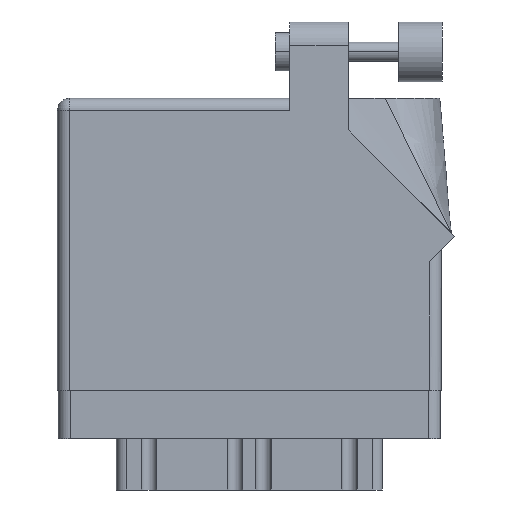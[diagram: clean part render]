
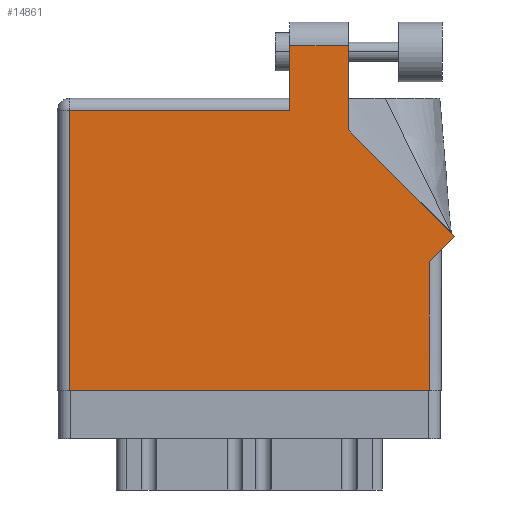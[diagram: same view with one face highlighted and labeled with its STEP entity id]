
A CAD part, front view. The second image highlights one B-rep face of the part: STEP entity #14861.
In plain terms, the highlighted face is planar.
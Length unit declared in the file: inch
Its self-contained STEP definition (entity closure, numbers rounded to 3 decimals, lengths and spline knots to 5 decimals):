
#793 = ORIENTED_EDGE ( 'NONE', *, *, #37293, .T. ) ;
#1068 = VECTOR ( 'NONE', #19315, 39.37008 ) ;
#1271 = PLANE ( 'NONE',  #6959 ) ;
#2713 = VECTOR ( 'NONE', #18833, 39.37008 ) ;
#2743 = CARTESIAN_POINT ( 'NONE',  ( 0.062, 0., 0. ) ) ;
#2892 = CARTESIAN_POINT ( 'NONE',  ( 1.948, 0., 0. ) ) ;
#3234 = VERTEX_POINT ( 'NONE', #12394 ) ;
#3263 = DIRECTION ( 'NONE',  ( -1., 0., 0. ) ) ;
#3584 = VECTOR ( 'NONE', #3263, 39.37008 ) ;
#3685 = EDGE_CURVE ( 'NONE', #7406, #26864, #22267, .T. ) ;
#4412 = CARTESIAN_POINT ( 'NONE',  ( 2.08071, 0.80771, 0. ) ) ;
#4518 = LINE ( 'NONE', #28428, #2713 ) ;
#6959 = AXIS2_PLACEMENT_3D ( 'NONE', #7171, #9752, #21686 ) ;
#6985 = CARTESIAN_POINT ( 'NONE',  ( 1.524, 1.805, 0. ) ) ;
#7171 = CARTESIAN_POINT ( 'NONE',  ( 0., 1.53, 0. ) ) ;
#7406 = VERTEX_POINT ( 'NONE', #2892 ) ;
#7435 = EDGE_CURVE ( 'NONE', #16643, #3234, #27183, .T. ) ;
#9401 = DIRECTION ( 'NONE',  ( 0., -1., 0. ) ) ;
#9676 = VERTEX_POINT ( 'NONE', #10788 ) ;
#9752 = DIRECTION ( 'NONE',  ( 0., 0., -1. ) ) ;
#9980 = EDGE_CURVE ( 'NONE', #36899, #30317, #17829, .T. ) ;
#10038 = ORIENTED_EDGE ( 'NONE', *, *, #17432, .T. ) ;
#10179 = VECTOR ( 'NONE', #17977, 39.37008 ) ;
#10788 = CARTESIAN_POINT ( 'NONE',  ( 2.08071, 0.80771, 0. ) ) ;
#11109 = CARTESIAN_POINT ( 'NONE',  ( 1.948, 0.737, 0. ) ) ;
#11259 = EDGE_CURVE ( 'NONE', #3234, #19204, #32910, .T. ) ;
#11352 = VECTOR ( 'NONE', #29773, 39.37008 ) ;
#11795 = CARTESIAN_POINT ( 'NONE',  ( 1.217, 1.468, 0. ) ) ;
#12394 = CARTESIAN_POINT ( 'NONE',  ( 0.062, 1.468, 0. ) ) ;
#12855 = LINE ( 'NONE', #4412, #1068 ) ;
#13798 = VECTOR ( 'NONE', #32057, 39.37008 ) ;
#14247 = EDGE_CURVE ( 'NONE', #30317, #24032, #20566, .T. ) ;
#14861 = ADVANCED_FACE ( 'NONE', ( #21871 ), #1271, .F. ) ;
#16643 = VERTEX_POINT ( 'NONE', #11795 ) ;
#16920 = EDGE_CURVE ( 'NONE', #26864, #9676, #32847, .T. ) ;
#17141 = VECTOR ( 'NONE', #17505, 39.37008 ) ;
#17432 = EDGE_CURVE ( 'NONE', #19204, #7406, #4518, .T. ) ;
#17505 = DIRECTION ( 'NONE',  ( 0., -1., 0. ) ) ;
#17627 = CARTESIAN_POINT ( 'NONE',  ( 1.217, 1.805, 0. ) ) ;
#17829 = LINE ( 'NONE', #21326, #11352 ) ;
#17896 = LINE ( 'NONE', #36609, #17141 ) ;
#17977 = DIRECTION ( 'NONE',  ( 0.707, 0.707, 0. ) ) ;
#17988 = CARTESIAN_POINT ( 'NONE',  ( 0., 1.468, 0. ) ) ;
#18727 = VECTOR ( 'NONE', #9401, 39.37008 ) ;
#18833 = DIRECTION ( 'NONE',  ( 1., 0., 0. ) ) ;
#19204 = VERTEX_POINT ( 'NONE', #28458 ) ;
#19315 = DIRECTION ( 'NONE',  ( -0.707, 0.707, 0. ) ) ;
#19731 = ORIENTED_EDGE ( 'NONE', *, *, #9980, .T. ) ;
#19830 = VECTOR ( 'NONE', #29573, 39.37008 ) ;
#20566 = LINE ( 'NONE', #17627, #19830 ) ;
#21326 = CARTESIAN_POINT ( 'NONE',  ( 1.524, 1.36442, 0. ) ) ;
#21686 = DIRECTION ( 'NONE',  ( -1., 0., 0. ) ) ;
#21871 = FACE_OUTER_BOUND ( 'NONE', #36660, .T. ) ;
#22267 = LINE ( 'NONE', #11109, #13798 ) ;
#22998 = CARTESIAN_POINT ( 'NONE',  ( 1.217, 1.805, 0. ) ) ;
#24032 = VERTEX_POINT ( 'NONE', #22998 ) ;
#24118 = EDGE_CURVE ( 'NONE', #24032, #16643, #17896, .T. ) ;
#24464 = CARTESIAN_POINT ( 'NONE',  ( 1.524, 1.36442, 0. ) ) ;
#24467 = ORIENTED_EDGE ( 'NONE', *, *, #16920, .T. ) ;
#26864 = VERTEX_POINT ( 'NONE', #31203 ) ;
#27183 = LINE ( 'NONE', #17988, #3584 ) ;
#28428 = CARTESIAN_POINT ( 'NONE',  ( 0., 0., 0. ) ) ;
#28458 = CARTESIAN_POINT ( 'NONE',  ( 0.062, 0., 0. ) ) ;
#29552 = ORIENTED_EDGE ( 'NONE', *, *, #7435, .T. ) ;
#29573 = DIRECTION ( 'NONE',  ( -1., 0., 0. ) ) ;
#29773 = DIRECTION ( 'NONE',  ( 0., 1., 0. ) ) ;
#29928 = ORIENTED_EDGE ( 'NONE', *, *, #3685, .T. ) ;
#30317 = VERTEX_POINT ( 'NONE', #6985 ) ;
#31203 = CARTESIAN_POINT ( 'NONE',  ( 1.948, 0.675, 0. ) ) ;
#31749 = CARTESIAN_POINT ( 'NONE',  ( 2.01, 0.737, 0. ) ) ;
#32057 = DIRECTION ( 'NONE',  ( 0., 1., 0. ) ) ;
#32847 = LINE ( 'NONE', #31749, #10179 ) ;
#32910 = LINE ( 'NONE', #2743, #18727 ) ;
#34506 = ORIENTED_EDGE ( 'NONE', *, *, #24118, .T. ) ;
#36231 = ORIENTED_EDGE ( 'NONE', *, *, #11259, .T. ) ;
#36232 = ORIENTED_EDGE ( 'NONE', *, *, #14247, .T. ) ;
#36609 = CARTESIAN_POINT ( 'NONE',  ( 1.217, 1.53, 0. ) ) ;
#36660 = EDGE_LOOP ( 'NONE', ( #19731, #36232, #34506, #29552, #36231, #10038, #29928, #24467, #793 ) ) ;
#36899 = VERTEX_POINT ( 'NONE', #24464 ) ;
#37293 = EDGE_CURVE ( 'NONE', #9676, #36899, #12855, .T. ) ;
